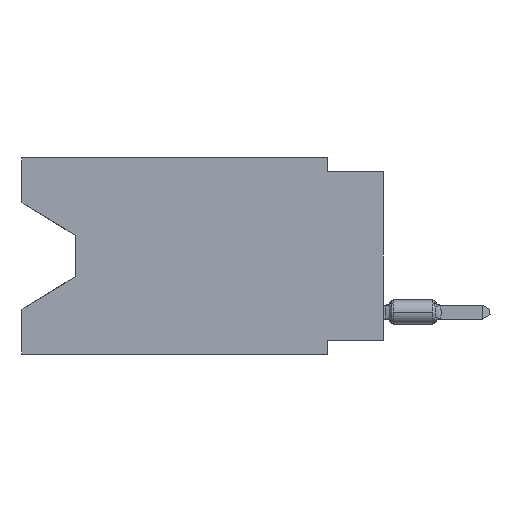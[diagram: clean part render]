
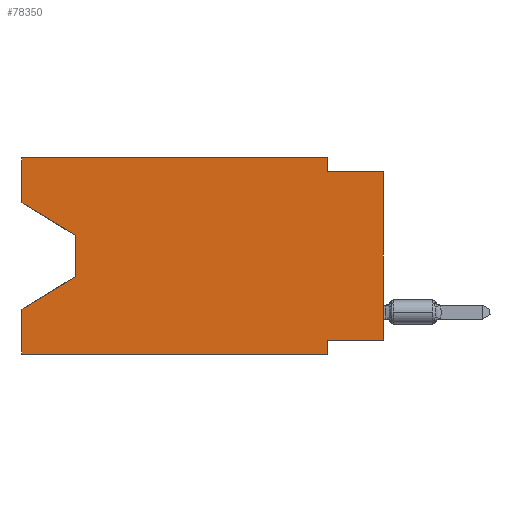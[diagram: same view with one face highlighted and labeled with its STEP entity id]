
A CAD part, left-side view. The second image highlights one B-rep face of the part: STEP entity #78350.
In plain terms, the highlighted planar face has unit normal (-1, 0, 0).
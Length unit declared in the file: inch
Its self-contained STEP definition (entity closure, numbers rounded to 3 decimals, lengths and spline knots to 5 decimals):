
#1428 = EDGE_CURVE ( 'NONE', #45111, #72289, #22000, .T. ) ;
#2075 = DIRECTION ( 'NONE',  ( 0., 0., -1. ) ) ;
#3305 = VECTOR ( 'NONE', #12642, 39.37008 ) ;
#6025 = CARTESIAN_POINT ( 'NONE',  ( 0., 0., -0.325 ) ) ;
#8035 = DIRECTION ( 'NONE',  ( 0., -1., 0. ) ) ;
#8334 = EDGE_CURVE ( 'NONE', #34222, #59793, #44488, .T. ) ;
#9036 = DIRECTION ( 'NONE',  ( 0., -1., 0. ) ) ;
#10691 = VERTEX_POINT ( 'NONE', #6025 ) ;
#11871 = EDGE_CURVE ( 'NONE', #57506, #45111, #18121, .T. ) ;
#12009 = CARTESIAN_POINT ( 'NONE',  ( 0., 0.645, 0. ) ) ;
#12642 = DIRECTION ( 'NONE',  ( 0., 1., 0. ) ) ;
#15100 = CARTESIAN_POINT ( 'NONE',  ( 0., 0.1, -0.35 ) ) ;
#17487 = VERTEX_POINT ( 'NONE', #79045 ) ;
#18121 = LINE ( 'NONE', #58416, #55500 ) ;
#18979 = DIRECTION ( 'NONE',  ( 0., 0.855, -0.519 ) ) ;
#21018 = CARTESIAN_POINT ( 'NONE',  ( 0., 0.1, -0.325 ) ) ;
#21837 = DIRECTION ( 'NONE',  ( 0., 0., 1. ) ) ;
#21875 = LINE ( 'NONE', #48888, #39288 ) ;
#22000 = LINE ( 'NONE', #49016, #24869 ) ;
#22599 = ORIENTED_EDGE ( 'NONE', *, *, #75389, .F. ) ;
#23673 = CARTESIAN_POINT ( 'NONE',  ( 0., 0.1, 0. ) ) ;
#23887 = DIRECTION ( 'NONE',  ( 0., -1., 0. ) ) ;
#23895 = ORIENTED_EDGE ( 'NONE', *, *, #32107, .T. ) ;
#24136 = DIRECTION ( 'NONE',  ( 0., 0., 1. ) ) ;
#24869 = VECTOR ( 'NONE', #2075, 39.37008 ) ;
#29908 = ORIENTED_EDGE ( 'NONE', *, *, #50509, .T. ) ;
#30438 = ORIENTED_EDGE ( 'NONE', *, *, #11871, .F. ) ;
#30977 = ORIENTED_EDGE ( 'NONE', *, *, #65000, .T. ) ;
#31289 = VERTEX_POINT ( 'NONE', #21018 ) ;
#32107 = EDGE_CURVE ( 'NONE', #56979, #17487, #53394, .T. ) ;
#32570 = EDGE_CURVE ( 'NONE', #50594, #56979, #74509, .T. ) ;
#32929 = DIRECTION ( 'NONE',  ( 0., -0.855, -0.519 ) ) ;
#34012 = LINE ( 'NONE', #79678, #60263 ) ;
#34222 = VERTEX_POINT ( 'NONE', #73139 ) ;
#35209 = CARTESIAN_POINT ( 'NONE',  ( 0., 0.55, -0.138 ) ) ;
#35550 = LINE ( 'NONE', #55487, #70569 ) ;
#35635 = EDGE_CURVE ( 'NONE', #72289, #78740, #49201, .T. ) ;
#37203 = VERTEX_POINT ( 'NONE', #15100 ) ;
#37901 = VECTOR ( 'NONE', #9036, 39.37008 ) ;
#39288 = VECTOR ( 'NONE', #61263, 39.37008 ) ;
#40220 = DIRECTION ( 'NONE',  ( 0., 0., -1. ) ) ;
#40572 = ORIENTED_EDGE ( 'NONE', *, *, #35635, .F. ) ;
#40785 = ORIENTED_EDGE ( 'NONE', *, *, #75464, .T. ) ;
#42327 = EDGE_LOOP ( 'NONE', ( #65991, #23895, #30977, #84301, #40785, #82893, #80777, #29908, #40572, #55960, #30438, #22599 ) ) ;
#42335 = EDGE_CURVE ( 'NONE', #10691, #31289, #57394, .T. ) ;
#42424 = VECTOR ( 'NONE', #8035, 39.37008 ) ;
#42674 = LINE ( 'NONE', #69668, #37901 ) ;
#44488 = LINE ( 'NONE', #76509, #58356 ) ;
#45111 = VERTEX_POINT ( 'NONE', #23673 ) ;
#46521 = FACE_OUTER_BOUND ( 'NONE', #42327, .T. ) ;
#48888 = CARTESIAN_POINT ( 'NONE',  ( 0., 0.645, 0. ) ) ;
#49016 = CARTESIAN_POINT ( 'NONE',  ( 0., 0.1, 0. ) ) ;
#49128 = VECTOR ( 'NONE', #32929, 39.37008 ) ;
#49201 = LINE ( 'NONE', #76193, #42424 ) ;
#50509 = EDGE_CURVE ( 'NONE', #10691, #78740, #35550, .T. ) ;
#50594 = VERTEX_POINT ( 'NONE', #74303 ) ;
#53364 = CARTESIAN_POINT ( 'NONE',  ( 0., 0., -0.325 ) ) ;
#53394 = LINE ( 'NONE', #68411, #84469 ) ;
#54614 = EDGE_CURVE ( 'NONE', #31289, #37203, #34012, .T. ) ;
#55487 = CARTESIAN_POINT ( 'NONE',  ( 0., 0., 0. ) ) ;
#55500 = VECTOR ( 'NONE', #23887, 39.37008 ) ;
#55960 = ORIENTED_EDGE ( 'NONE', *, *, #1428, .F. ) ;
#56979 = VERTEX_POINT ( 'NONE', #35209 ) ;
#57394 = LINE ( 'NONE', #53364, #3305 ) ;
#57506 = VERTEX_POINT ( 'NONE', #70378 ) ;
#58356 = VECTOR ( 'NONE', #24136, 39.37008 ) ;
#58416 = CARTESIAN_POINT ( 'NONE',  ( 0., 0.645, 0. ) ) ;
#59374 = PLANE ( 'NONE',  #80112 ) ;
#59793 = VERTEX_POINT ( 'NONE', #67720 ) ;
#60263 = VECTOR ( 'NONE', #40220, 39.37008 ) ;
#61263 = DIRECTION ( 'NONE',  ( 0., 0., 1. ) ) ;
#65000 = EDGE_CURVE ( 'NONE', #17487, #59793, #78341, .T. ) ;
#65100 = VECTOR ( 'NONE', #18979, 39.37008 ) ;
#65991 = ORIENTED_EDGE ( 'NONE', *, *, #32570, .T. ) ;
#67099 = DIRECTION ( 'NONE',  ( 0., 0., -1. ) ) ;
#67720 = CARTESIAN_POINT ( 'NONE',  ( 0., 0.645, -0.26975 ) ) ;
#67862 = CARTESIAN_POINT ( 'NONE',  ( 0., 0.645, -0.08025 ) ) ;
#68411 = CARTESIAN_POINT ( 'NONE',  ( 0., 0.55, -0.138 ) ) ;
#69668 = CARTESIAN_POINT ( 'NONE',  ( 0., 0.645, -0.35 ) ) ;
#70378 = CARTESIAN_POINT ( 'NONE',  ( 0., 0.645, 0. ) ) ;
#70569 = VECTOR ( 'NONE', #21837, 39.37008 ) ;
#72289 = VERTEX_POINT ( 'NONE', #86057 ) ;
#73101 = DIRECTION ( 'NONE',  ( 0., 0., -1. ) ) ;
#73139 = CARTESIAN_POINT ( 'NONE',  ( 0., 0.645, -0.35 ) ) ;
#74303 = CARTESIAN_POINT ( 'NONE',  ( 0., 0.645, -0.08025 ) ) ;
#74509 = LINE ( 'NONE', #67862, #49128 ) ;
#75389 = EDGE_CURVE ( 'NONE', #50594, #57506, #21875, .T. ) ;
#75464 = EDGE_CURVE ( 'NONE', #34222, #37203, #42674, .T. ) ;
#76193 = CARTESIAN_POINT ( 'NONE',  ( 0., 0., -0.025 ) ) ;
#76509 = CARTESIAN_POINT ( 'NONE',  ( 0., 0.645, 0. ) ) ;
#77012 = CARTESIAN_POINT ( 'NONE',  ( 0., 0., -0.025 ) ) ;
#78341 = LINE ( 'NONE', #79655, #65100 ) ;
#78350 = ADVANCED_FACE ( 'NONE', ( #46521 ), #59374, .F. ) ;
#78740 = VERTEX_POINT ( 'NONE', #77012 ) ;
#79045 = CARTESIAN_POINT ( 'NONE',  ( 0., 0.55, -0.212 ) ) ;
#79321 = DIRECTION ( 'NONE',  ( 1., 0., 0. ) ) ;
#79655 = CARTESIAN_POINT ( 'NONE',  ( 0., 0.55, -0.212 ) ) ;
#79678 = CARTESIAN_POINT ( 'NONE',  ( 0., 0.1, -0.35 ) ) ;
#80112 = AXIS2_PLACEMENT_3D ( 'NONE', #12009, #79321, #73101 ) ;
#80777 = ORIENTED_EDGE ( 'NONE', *, *, #42335, .F. ) ;
#82893 = ORIENTED_EDGE ( 'NONE', *, *, #54614, .F. ) ;
#84301 = ORIENTED_EDGE ( 'NONE', *, *, #8334, .F. ) ;
#84469 = VECTOR ( 'NONE', #67099, 39.37008 ) ;
#86057 = CARTESIAN_POINT ( 'NONE',  ( 0., 0.1, -0.025 ) ) ;
